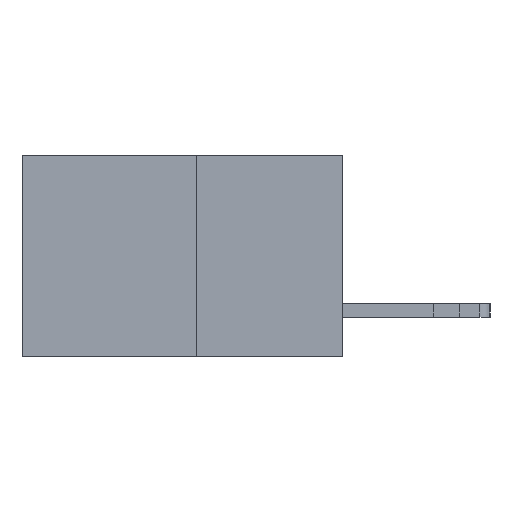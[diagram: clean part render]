
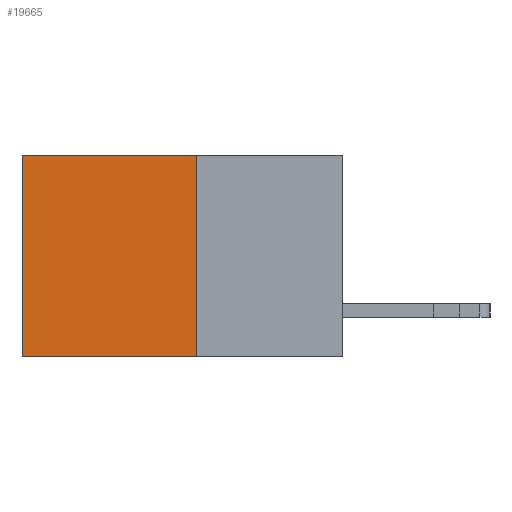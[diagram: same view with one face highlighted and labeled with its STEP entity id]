
A CAD part, left-side view. The second image highlights one B-rep face of the part: STEP entity #19665.
In plain terms, the highlighted planar face has unit normal (-1, 0, 0).
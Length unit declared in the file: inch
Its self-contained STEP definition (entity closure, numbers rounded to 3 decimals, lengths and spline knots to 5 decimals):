
#854 = ORIENTED_EDGE ( 'NONE', *, *, #18457, .F. ) ;
#1868 = FACE_OUTER_BOUND ( 'NONE', #14525, .T. ) ;
#2902 = LINE ( 'NONE', #19347, #19041 ) ;
#3454 = LINE ( 'NONE', #4150, #19579 ) ;
#3985 = VERTEX_POINT ( 'NONE', #5517 ) ;
#4150 = CARTESIAN_POINT ( 'NONE',  ( 0.277, 0.59, -0.37 ) ) ;
#4938 = VECTOR ( 'NONE', #5930, 39.37008 ) ;
#4981 = AXIS2_PLACEMENT_3D ( 'NONE', #17558, #8184, #19119 ) ;
#5517 = CARTESIAN_POINT ( 'NONE',  ( 0.277, 0.27, -0.37 ) ) ;
#5930 = DIRECTION ( 'NONE',  ( 0., 1., 0. ) ) ;
#6336 = EDGE_CURVE ( 'NONE', #8660, #3985, #12909, .T. ) ;
#6616 = ORIENTED_EDGE ( 'NONE', *, *, #8485, .T. ) ;
#6624 = CARTESIAN_POINT ( 'NONE',  ( 0.277, 0.59, -0.37 ) ) ;
#6814 = DIRECTION ( 'NONE',  ( 0., 1., 0. ) ) ;
#7693 = VERTEX_POINT ( 'NONE', #6624 ) ;
#8129 = DIRECTION ( 'NONE',  ( 0., 0., -1. ) ) ;
#8184 = DIRECTION ( 'NONE',  ( 1., 0., 0. ) ) ;
#8485 = EDGE_CURVE ( 'NONE', #8660, #10012, #12296, .T. ) ;
#8660 = VERTEX_POINT ( 'NONE', #18869 ) ;
#8721 = VECTOR ( 'NONE', #8129, 39.37008 ) ;
#10012 = VERTEX_POINT ( 'NONE', #12972 ) ;
#10446 = DIRECTION ( 'NONE',  ( 0., 0., -1. ) ) ;
#10498 = ORIENTED_EDGE ( 'NONE', *, *, #6336, .F. ) ;
#12246 = CARTESIAN_POINT ( 'NONE',  ( 0.277, 0.27, 0. ) ) ;
#12296 = LINE ( 'NONE', #12246, #4938 ) ;
#12909 = LINE ( 'NONE', #19061, #8721 ) ;
#12972 = CARTESIAN_POINT ( 'NONE',  ( 0.277, 0.59, 0. ) ) ;
#13445 = ORIENTED_EDGE ( 'NONE', *, *, #17118, .T. ) ;
#14525 = EDGE_LOOP ( 'NONE', ( #13445, #854, #10498, #6616 ) ) ;
#15781 = PLANE ( 'NONE',  #4981 ) ;
#17118 = EDGE_CURVE ( 'NONE', #10012, #7693, #3454, .T. ) ;
#17558 = CARTESIAN_POINT ( 'NONE',  ( 0.277, 0.27, -0.37 ) ) ;
#18457 = EDGE_CURVE ( 'NONE', #3985, #7693, #2902, .T. ) ;
#18869 = CARTESIAN_POINT ( 'NONE',  ( 0.277, 0.27, 0. ) ) ;
#19041 = VECTOR ( 'NONE', #6814, 39.37008 ) ;
#19061 = CARTESIAN_POINT ( 'NONE',  ( 0.277, 0.27, -0.37 ) ) ;
#19119 = DIRECTION ( 'NONE',  ( 0., 0., -1. ) ) ;
#19347 = CARTESIAN_POINT ( 'NONE',  ( 0.277, 0.27, -0.37 ) ) ;
#19579 = VECTOR ( 'NONE', #10446, 39.37008 ) ;
#19665 = ADVANCED_FACE ( 'NONE', ( #1868 ), #15781, .F. ) ;
